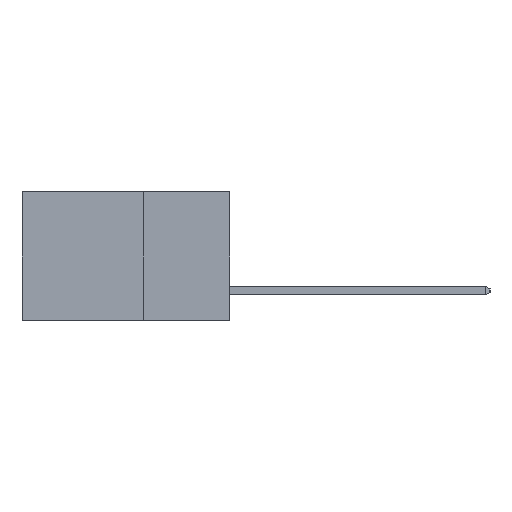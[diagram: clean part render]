
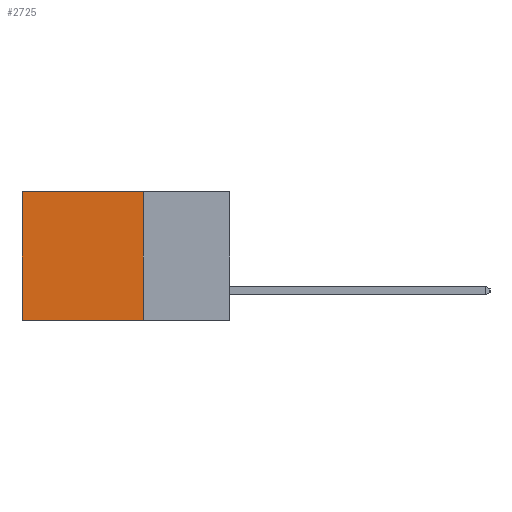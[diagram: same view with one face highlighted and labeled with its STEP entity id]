
A CAD part, left-side view. The second image highlights one B-rep face of the part: STEP entity #2725.
In plain terms, the highlighted planar face has unit normal (-1, 0, 0).
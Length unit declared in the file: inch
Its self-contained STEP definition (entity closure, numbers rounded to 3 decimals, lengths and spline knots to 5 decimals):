
#1235 = DIRECTION ( 'NONE',  ( 0., 0., -1. ) ) ;
#1333 = VERTEX_POINT ( 'NONE', #2981 ) ;
#1536 = LINE ( 'NONE', #11705, #13534 ) ;
#2145 = ORIENTED_EDGE ( 'NONE', *, *, #4571, .F. ) ;
#2213 = VERTEX_POINT ( 'NONE', #4901 ) ;
#2324 = EDGE_LOOP ( 'NONE', ( #4568, #4941, #2145, #14838 ) ) ;
#2698 = LINE ( 'NONE', #15047, #14592 ) ;
#2725 = ADVANCED_FACE ( 'NONE', ( #3132 ), #6680, .F. ) ;
#2981 = CARTESIAN_POINT ( 'NONE',  ( 0.2615, 0.6, -0.37 ) ) ;
#3079 = DIRECTION ( 'NONE',  ( 0., 1., 0. ) ) ;
#3132 = FACE_OUTER_BOUND ( 'NONE', #2324, .T. ) ;
#3435 = CARTESIAN_POINT ( 'NONE',  ( 0.2615, 0.25, 0. ) ) ;
#4233 = CARTESIAN_POINT ( 'NONE',  ( 0.2615, 0.25, -0.37 ) ) ;
#4568 = ORIENTED_EDGE ( 'NONE', *, *, #11994, .T. ) ;
#4571 = EDGE_CURVE ( 'NONE', #5483, #9285, #2698, .T. ) ;
#4901 = CARTESIAN_POINT ( 'NONE',  ( 0.2615, 0.6, 0. ) ) ;
#4941 = ORIENTED_EDGE ( 'NONE', *, *, #7699, .F. ) ;
#5366 = CARTESIAN_POINT ( 'NONE',  ( 0.2615, 0.25, -0.37 ) ) ;
#5483 = VERTEX_POINT ( 'NONE', #3435 ) ;
#6154 = DIRECTION ( 'NONE',  ( 1., 0., 0. ) ) ;
#6680 = PLANE ( 'NONE',  #14070 ) ;
#7299 = VECTOR ( 'NONE', #3079, 39.37008 ) ;
#7659 = LINE ( 'NONE', #4233, #7299 ) ;
#7699 = EDGE_CURVE ( 'NONE', #9285, #1333, #7659, .T. ) ;
#9285 = VERTEX_POINT ( 'NONE', #11632 ) ;
#10615 = CARTESIAN_POINT ( 'NONE',  ( 0.2615, 0.6, -0.37 ) ) ;
#11231 = DIRECTION ( 'NONE',  ( 0., 0., -1. ) ) ;
#11632 = CARTESIAN_POINT ( 'NONE',  ( 0.2615, 0.25, -0.37 ) ) ;
#11705 = CARTESIAN_POINT ( 'NONE',  ( 0.2615, 0.25, 0. ) ) ;
#11871 = VECTOR ( 'NONE', #1235, 39.37008 ) ;
#11994 = EDGE_CURVE ( 'NONE', #2213, #1333, #14821, .T. ) ;
#12859 = DIRECTION ( 'NONE',  ( 0., 1., 0. ) ) ;
#13534 = VECTOR ( 'NONE', #12859, 39.37008 ) ;
#14070 = AXIS2_PLACEMENT_3D ( 'NONE', #5366, #6154, #11231 ) ;
#14403 = EDGE_CURVE ( 'NONE', #5483, #2213, #1536, .T. ) ;
#14535 = DIRECTION ( 'NONE',  ( 0., 0., -1. ) ) ;
#14592 = VECTOR ( 'NONE', #14535, 39.37008 ) ;
#14821 = LINE ( 'NONE', #10615, #11871 ) ;
#14838 = ORIENTED_EDGE ( 'NONE', *, *, #14403, .T. ) ;
#15047 = CARTESIAN_POINT ( 'NONE',  ( 0.2615, 0.25, -0.37 ) ) ;
